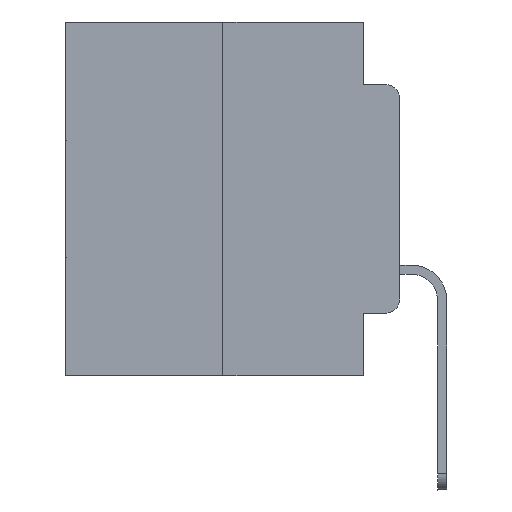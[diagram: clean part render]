
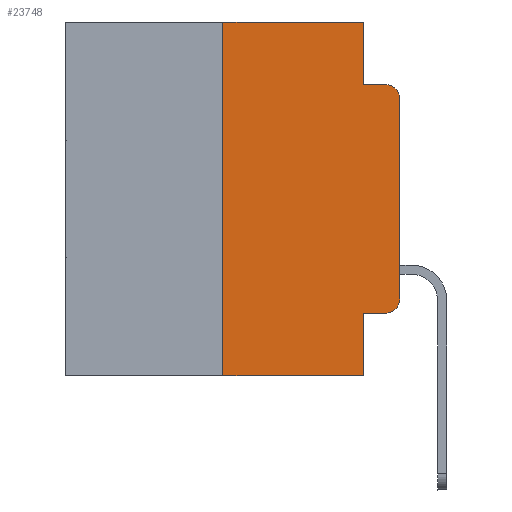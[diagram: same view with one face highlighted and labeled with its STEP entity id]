
A CAD part, left-side view. The second image highlights one B-rep face of the part: STEP entity #23748.
In plain terms, the highlighted planar face has unit normal (-1, 0, 0).
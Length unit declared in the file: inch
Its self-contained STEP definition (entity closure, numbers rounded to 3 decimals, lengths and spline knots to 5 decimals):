
#596 = CARTESIAN_POINT ( 'NONE',  ( 0., 0.051, -0.0885 ) ) ;
#752 = CARTESIAN_POINT ( 'NONE',  ( 0., 0.02, -0.3915 ) ) ;
#1038 = CARTESIAN_POINT ( 'NONE',  ( 0., 0.051, -0.4115 ) ) ;
#1355 = ORIENTED_EDGE ( 'NONE', *, *, #22280, .F. ) ;
#1386 = CARTESIAN_POINT ( 'NONE',  ( 0., 0.051, 0. ) ) ;
#2192 = EDGE_CURVE ( 'NONE', #13773, #4401, #22722, .T. ) ;
#2297 = ORIENTED_EDGE ( 'NONE', *, *, #18516, .F. ) ;
#2450 = CARTESIAN_POINT ( 'NONE',  ( 0., 0.02, -0.1085 ) ) ;
#2565 = ORIENTED_EDGE ( 'NONE', *, *, #13232, .T. ) ;
#2986 = EDGE_CURVE ( 'NONE', #10976, #8353, #7612, .T. ) ;
#3002 = DIRECTION ( 'NONE',  ( 0., -1., 0. ) ) ;
#3423 = PLANE ( 'NONE',  #14608 ) ;
#3460 = LINE ( 'NONE', #5696, #5689 ) ;
#3910 = VERTEX_POINT ( 'NONE', #17932 ) ;
#3921 = VECTOR ( 'NONE', #3002, 39.37008 ) ;
#4401 = VERTEX_POINT ( 'NONE', #5922 ) ;
#4781 = VERTEX_POINT ( 'NONE', #13946 ) ;
#5689 = VECTOR ( 'NONE', #20846, 39.37008 ) ;
#5696 = CARTESIAN_POINT ( 'NONE',  ( 0., 0.051, 0. ) ) ;
#5922 = CARTESIAN_POINT ( 'NONE',  ( 0., 0.02, -0.0885 ) ) ;
#6047 = VECTOR ( 'NONE', #23932, 39.37008 ) ;
#6341 = VERTEX_POINT ( 'NONE', #24202 ) ;
#6380 = ORIENTED_EDGE ( 'NONE', *, *, #13422, .T. ) ;
#7090 = EDGE_LOOP ( 'NONE', ( #10139, #2565, #26372, #16587, #1355, #17333, #18618, #2297, #6380, #19246 ) ) ;
#7190 = CARTESIAN_POINT ( 'NONE',  ( 0., 0.473, -0.5 ) ) ;
#7612 = LINE ( 'NONE', #7190, #3921 ) ;
#7817 = VECTOR ( 'NONE', #16138, 39.37008 ) ;
#8188 = LINE ( 'NONE', #21099, #23191 ) ;
#8353 = VERTEX_POINT ( 'NONE', #12763 ) ;
#8598 = CARTESIAN_POINT ( 'NONE',  ( 0., 0.25, -0.5 ) ) ;
#8779 = DIRECTION ( 'NONE',  ( 0., 0., 1. ) ) ;
#9076 = VERTEX_POINT ( 'NONE', #13711 ) ;
#9292 = DIRECTION ( 'NONE',  ( -1., 0., 0. ) ) ;
#9433 = DIRECTION ( 'NONE',  ( 0., 0., 1. ) ) ;
#10139 = ORIENTED_EDGE ( 'NONE', *, *, #26071, .T. ) ;
#10952 = AXIS2_PLACEMENT_3D ( 'NONE', #2450, #17172, #15062 ) ;
#10976 = VERTEX_POINT ( 'NONE', #8598 ) ;
#11115 = CARTESIAN_POINT ( 'NONE',  ( 0., 0.25, 0. ) ) ;
#11955 = VECTOR ( 'NONE', #8779, 39.37008 ) ;
#12763 = CARTESIAN_POINT ( 'NONE',  ( 0., 0.051, -0.5 ) ) ;
#13232 = EDGE_CURVE ( 'NONE', #6341, #4401, #23076, .T. ) ;
#13422 = EDGE_CURVE ( 'NONE', #4781, #3910, #17590, .T. ) ;
#13711 = CARTESIAN_POINT ( 'NONE',  ( 0., 0.051, 0. ) ) ;
#13763 = CARTESIAN_POINT ( 'NONE',  ( 0., 0.473, 0. ) ) ;
#13773 = VERTEX_POINT ( 'NONE', #596 ) ;
#13946 = CARTESIAN_POINT ( 'NONE',  ( 0., 0.051, -0.4115 ) ) ;
#14096 = CIRCLE ( 'NONE', #21720, 0.02 ) ;
#14608 = AXIS2_PLACEMENT_3D ( 'NONE', #20542, #23628, #23758 ) ;
#15062 = DIRECTION ( 'NONE',  ( 0., 0., -1. ) ) ;
#16138 = DIRECTION ( 'NONE',  ( 0., -1., 0. ) ) ;
#16267 = LINE ( 'NONE', #1386, #27594 ) ;
#16587 = ORIENTED_EDGE ( 'NONE', *, *, #24513, .F. ) ;
#16820 = VERTEX_POINT ( 'NONE', #11115 ) ;
#17172 = DIRECTION ( 'NONE',  ( -1., 0., 0. ) ) ;
#17333 = ORIENTED_EDGE ( 'NONE', *, *, #26641, .F. ) ;
#17590 = LINE ( 'NONE', #1038, #6047 ) ;
#17855 = DIRECTION ( 'NONE',  ( 0., 0., -1. ) ) ;
#17932 = CARTESIAN_POINT ( 'NONE',  ( 0., 0.02, -0.4115 ) ) ;
#18010 = EDGE_CURVE ( 'NONE', #3910, #26323, #14096, .T. ) ;
#18516 = EDGE_CURVE ( 'NONE', #4781, #8353, #16267, .T. ) ;
#18618 = ORIENTED_EDGE ( 'NONE', *, *, #2986, .T. ) ;
#19246 = ORIENTED_EDGE ( 'NONE', *, *, #18010, .T. ) ;
#19590 = CARTESIAN_POINT ( 'NONE',  ( 0., 0., -0.3915 ) ) ;
#20072 = LINE ( 'NONE', #24440, #11955 ) ;
#20542 = CARTESIAN_POINT ( 'NONE',  ( 0., 0.473, 0. ) ) ;
#20623 = LINE ( 'NONE', #13763, #7817 ) ;
#20846 = DIRECTION ( 'NONE',  ( 0., 0., -1. ) ) ;
#21099 = CARTESIAN_POINT ( 'NONE',  ( 0., 0.25, 0. ) ) ;
#21720 = AXIS2_PLACEMENT_3D ( 'NONE', #752, #9292, #17855 ) ;
#22003 = VECTOR ( 'NONE', #22584, 39.37008 ) ;
#22280 = EDGE_CURVE ( 'NONE', #16820, #9076, #20623, .T. ) ;
#22584 = DIRECTION ( 'NONE',  ( 0., -1., 0. ) ) ;
#22661 = FACE_OUTER_BOUND ( 'NONE', #7090, .T. ) ;
#22722 = LINE ( 'NONE', #24691, #22003 ) ;
#23076 = CIRCLE ( 'NONE', #10952, 0.02 ) ;
#23191 = VECTOR ( 'NONE', #9433, 39.37008 ) ;
#23628 = DIRECTION ( 'NONE',  ( 1., 0., 0. ) ) ;
#23748 = ADVANCED_FACE ( 'NONE', ( #22661 ), #3423, .F. ) ;
#23758 = DIRECTION ( 'NONE',  ( 0., 0., -1. ) ) ;
#23932 = DIRECTION ( 'NONE',  ( 0., -1., 0. ) ) ;
#24202 = CARTESIAN_POINT ( 'NONE',  ( 0., 0., -0.1085 ) ) ;
#24440 = CARTESIAN_POINT ( 'NONE',  ( 0., 0., 0. ) ) ;
#24513 = EDGE_CURVE ( 'NONE', #9076, #13773, #3460, .T. ) ;
#24691 = CARTESIAN_POINT ( 'NONE',  ( 0., 0.051, -0.0885 ) ) ;
#24849 = DIRECTION ( 'NONE',  ( 0., 0., -1. ) ) ;
#26071 = EDGE_CURVE ( 'NONE', #26323, #6341, #20072, .T. ) ;
#26323 = VERTEX_POINT ( 'NONE', #19590 ) ;
#26372 = ORIENTED_EDGE ( 'NONE', *, *, #2192, .F. ) ;
#26641 = EDGE_CURVE ( 'NONE', #10976, #16820, #8188, .T. ) ;
#27594 = VECTOR ( 'NONE', #24849, 39.37008 ) ;
